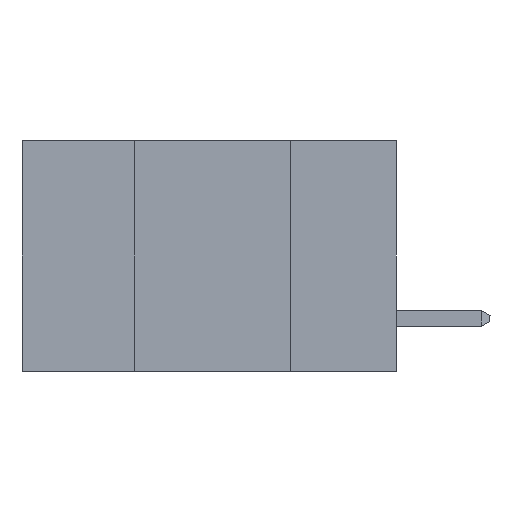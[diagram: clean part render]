
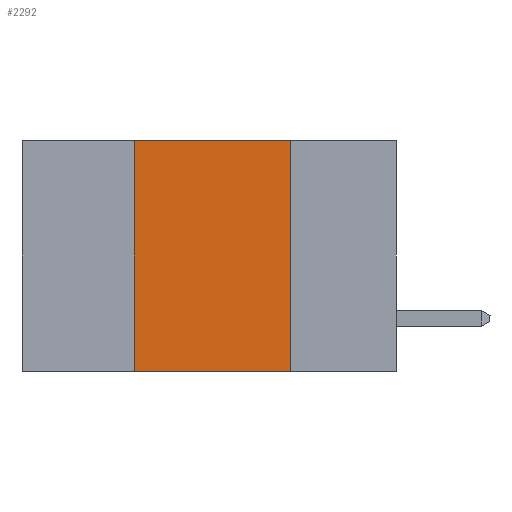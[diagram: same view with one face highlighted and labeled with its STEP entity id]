
A CAD part, left-side view. The second image highlights one B-rep face of the part: STEP entity #2292.
In plain terms, the highlighted planar face has unit normal (-1, 0, 0).
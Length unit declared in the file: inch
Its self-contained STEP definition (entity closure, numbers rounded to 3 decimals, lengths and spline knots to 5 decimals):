
#581 = CARTESIAN_POINT ( 'NONE',  ( 0., 0.6, 0. ) ) ;
#651 = CARTESIAN_POINT ( 'NONE',  ( 0., 0.17, -0.37 ) ) ;
#778 = LINE ( 'NONE', #15152, #4828 ) ;
#1094 = EDGE_CURVE ( 'NONE', #14974, #10903, #7131, .T. ) ;
#2113 = CARTESIAN_POINT ( 'NONE',  ( 0., 0.42, -0.37 ) ) ;
#2292 = ADVANCED_FACE ( 'NONE', ( #16462 ), #12162, .F. ) ;
#2314 = VERTEX_POINT ( 'NONE', #7334 ) ;
#2401 = ORIENTED_EDGE ( 'NONE', *, *, #1094, .F. ) ;
#2842 = CARTESIAN_POINT ( 'NONE',  ( 0., 0.17, 0. ) ) ;
#3463 = VECTOR ( 'NONE', #8983, 39.37008 ) ;
#3467 = EDGE_CURVE ( 'NONE', #13251, #2314, #7260, .T. ) ;
#3588 = VECTOR ( 'NONE', #15946, 39.37008 ) ;
#3874 = ORIENTED_EDGE ( 'NONE', *, *, #16768, .T. ) ;
#4828 = VECTOR ( 'NONE', #8381, 39.37008 ) ;
#7131 = LINE ( 'NONE', #11668, #3463 ) ;
#7260 = LINE ( 'NONE', #16514, #3588 ) ;
#7334 = CARTESIAN_POINT ( 'NONE',  ( 0., 0.42, 0. ) ) ;
#7468 = DIRECTION ( 'NONE',  ( 0., -1., 0. ) ) ;
#7510 = LINE ( 'NONE', #16956, #11570 ) ;
#7999 = ORIENTED_EDGE ( 'NONE', *, *, #3467, .F. ) ;
#8381 = DIRECTION ( 'NONE',  ( 0., -1., 0. ) ) ;
#8983 = DIRECTION ( 'NONE',  ( 0., 0., -1. ) ) ;
#10237 = EDGE_LOOP ( 'NONE', ( #2401, #15651, #7999, #3874 ) ) ;
#10903 = VERTEX_POINT ( 'NONE', #651 ) ;
#11570 = VECTOR ( 'NONE', #7468, 39.37008 ) ;
#11668 = CARTESIAN_POINT ( 'NONE',  ( 0., 0.17, -0.37 ) ) ;
#11986 = DIRECTION ( 'NONE',  ( 0., 0., -1. ) ) ;
#12070 = DIRECTION ( 'NONE',  ( 1., 0., 0. ) ) ;
#12162 = PLANE ( 'NONE',  #16108 ) ;
#12932 = EDGE_CURVE ( 'NONE', #2314, #14974, #778, .T. ) ;
#13251 = VERTEX_POINT ( 'NONE', #2113 ) ;
#14974 = VERTEX_POINT ( 'NONE', #2842 ) ;
#15152 = CARTESIAN_POINT ( 'NONE',  ( 0., 0.6, 0. ) ) ;
#15651 = ORIENTED_EDGE ( 'NONE', *, *, #12932, .F. ) ;
#15946 = DIRECTION ( 'NONE',  ( 0., 0., 1. ) ) ;
#16108 = AXIS2_PLACEMENT_3D ( 'NONE', #581, #12070, #11986 ) ;
#16462 = FACE_OUTER_BOUND ( 'NONE', #10237, .T. ) ;
#16514 = CARTESIAN_POINT ( 'NONE',  ( 0., 0.42, -0.37 ) ) ;
#16768 = EDGE_CURVE ( 'NONE', #13251, #10903, #7510, .T. ) ;
#16956 = CARTESIAN_POINT ( 'NONE',  ( 0., 0.6, -0.37 ) ) ;
